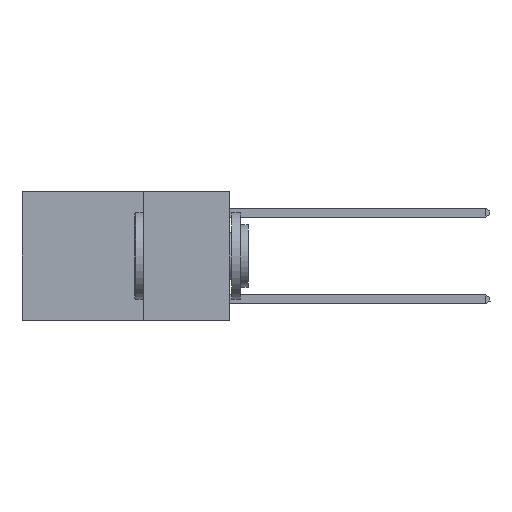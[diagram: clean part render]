
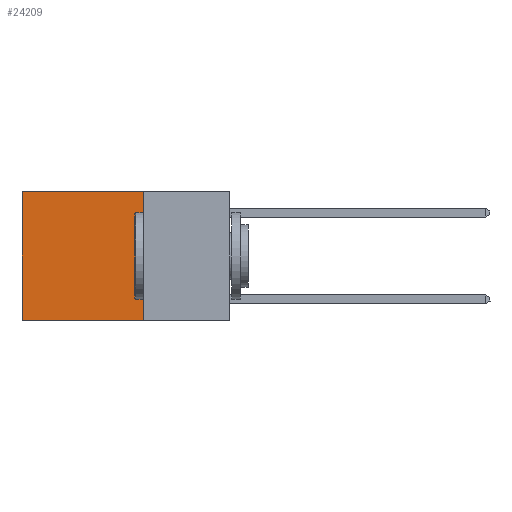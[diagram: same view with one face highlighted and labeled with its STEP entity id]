
A CAD part, left-side view. The second image highlights one B-rep face of the part: STEP entity #24209.
In plain terms, the highlighted planar face has unit normal (-1, 0, 0).
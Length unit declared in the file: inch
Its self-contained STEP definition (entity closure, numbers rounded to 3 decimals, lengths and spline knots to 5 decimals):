
#1020 = LINE ( 'NONE', #13423, #13299 ) ;
#1684 = CARTESIAN_POINT ( 'NONE',  ( 0.2625, 0.25, 0. ) ) ;
#1719 = VERTEX_POINT ( 'NONE', #13648 ) ;
#2318 = EDGE_CURVE ( 'NONE', #17988, #12172, #14155, .T. ) ;
#2426 = ORIENTED_EDGE ( 'NONE', *, *, #5654, .F. ) ;
#3230 = DIRECTION ( 'NONE',  ( 0., 0., -1. ) ) ;
#3799 = FACE_OUTER_BOUND ( 'NONE', #11900, .T. ) ;
#4474 = CARTESIAN_POINT ( 'NONE',  ( 0.2625, 0.25, 0. ) ) ;
#4949 = DIRECTION ( 'NONE',  ( 0., 1., 0. ) ) ;
#5654 = EDGE_CURVE ( 'NONE', #19329, #17988, #19392, .T. ) ;
#7287 = ORIENTED_EDGE ( 'NONE', *, *, #13122, .T. ) ;
#7885 = CARTESIAN_POINT ( 'NONE',  ( 0.2625, 0.25, -0.37 ) ) ;
#9170 = DIRECTION ( 'NONE',  ( 0., 0., -1. ) ) ;
#10114 = CARTESIAN_POINT ( 'NONE',  ( 0.2625, 0.25, -0.37 ) ) ;
#10671 = AXIS2_PLACEMENT_3D ( 'NONE', #1684, #16597, #3230 ) ;
#11012 = VECTOR ( 'NONE', #9170, 39.37008 ) ;
#11900 = EDGE_LOOP ( 'NONE', ( #7287, #24105, #2426, #12348 ) ) ;
#12172 = VERTEX_POINT ( 'NONE', #21401 ) ;
#12348 = ORIENTED_EDGE ( 'NONE', *, *, #16541, .T. ) ;
#12590 = VECTOR ( 'NONE', #22654, 39.37008 ) ;
#13122 = EDGE_CURVE ( 'NONE', #1719, #12172, #19864, .T. ) ;
#13299 = VECTOR ( 'NONE', #4949, 39.37008 ) ;
#13423 = CARTESIAN_POINT ( 'NONE',  ( 0.2625, 0.25, 0. ) ) ;
#13648 = CARTESIAN_POINT ( 'NONE',  ( 0.2625, 0.6, 0. ) ) ;
#14155 = LINE ( 'NONE', #10114, #12590 ) ;
#16541 = EDGE_CURVE ( 'NONE', #19329, #1719, #1020, .T. ) ;
#16597 = DIRECTION ( 'NONE',  ( 1., 0., 0. ) ) ;
#17988 = VERTEX_POINT ( 'NONE', #7885 ) ;
#19329 = VERTEX_POINT ( 'NONE', #4474 ) ;
#19384 = VECTOR ( 'NONE', #23295, 39.37008 ) ;
#19392 = LINE ( 'NONE', #25233, #19384 ) ;
#19864 = LINE ( 'NONE', #26024, #11012 ) ;
#20756 = PLANE ( 'NONE',  #10671 ) ;
#21401 = CARTESIAN_POINT ( 'NONE',  ( 0.2625, 0.6, -0.37 ) ) ;
#22654 = DIRECTION ( 'NONE',  ( 0., 1., 0. ) ) ;
#23295 = DIRECTION ( 'NONE',  ( 0., 0., -1. ) ) ;
#24105 = ORIENTED_EDGE ( 'NONE', *, *, #2318, .F. ) ;
#24209 = ADVANCED_FACE ( 'NONE', ( #3799 ), #20756, .F. ) ;
#25233 = CARTESIAN_POINT ( 'NONE',  ( 0.2625, 0.25, 0. ) ) ;
#26024 = CARTESIAN_POINT ( 'NONE',  ( 0.2625, 0.6, 0. ) ) ;
